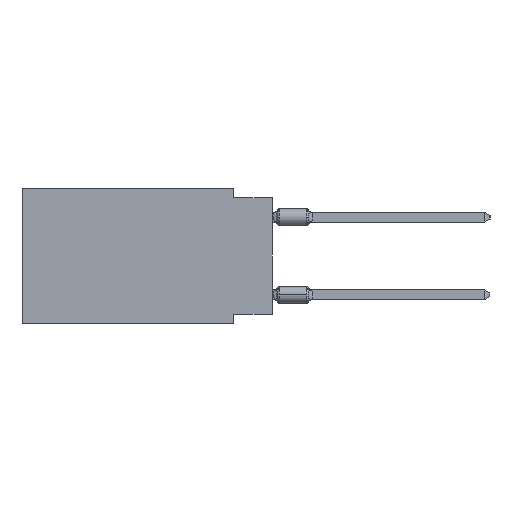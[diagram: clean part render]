
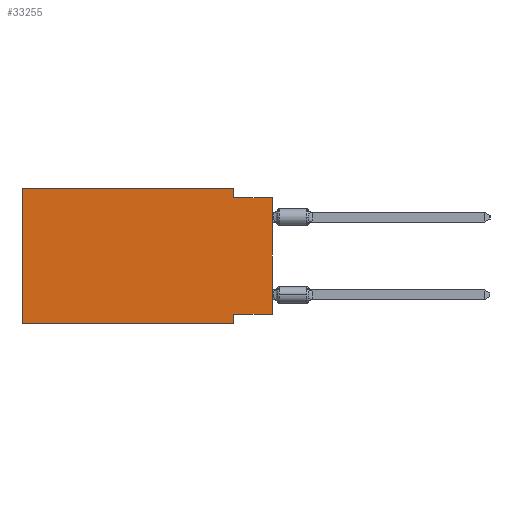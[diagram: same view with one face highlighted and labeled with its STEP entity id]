
A CAD part, left-side view. The second image highlights one B-rep face of the part: STEP entity #33255.
In plain terms, the highlighted planar face has unit normal (-1, 0, 0).
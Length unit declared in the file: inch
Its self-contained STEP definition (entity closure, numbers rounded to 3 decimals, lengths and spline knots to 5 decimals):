
#394 = CARTESIAN_POINT ( 'NONE',  ( 0., 0., -0.025 ) ) ;
#1127 = VERTEX_POINT ( 'NONE', #8704 ) ;
#1514 = EDGE_CURVE ( 'NONE', #1127, #52534, #60189, .T. ) ;
#3467 = VECTOR ( 'NONE', #20950, 39.37008 ) ;
#5479 = DIRECTION ( 'NONE',  ( 0., 0., -1. ) ) ;
#6096 = VECTOR ( 'NONE', #8203, 39.37008 ) ;
#6951 = EDGE_CURVE ( 'NONE', #21012, #21670, #28634, .T. ) ;
#8203 = DIRECTION ( 'NONE',  ( 0., 1., 0. ) ) ;
#8367 = CARTESIAN_POINT ( 'NONE',  ( 0., 0.1, -0.325 ) ) ;
#8704 = CARTESIAN_POINT ( 'NONE',  ( 0., 0.645, -0.35 ) ) ;
#10356 = VECTOR ( 'NONE', #22928, 39.37008 ) ;
#10448 = CARTESIAN_POINT ( 'NONE',  ( 0., 0.1, -0.35 ) ) ;
#11042 = DIRECTION ( 'NONE',  ( 0., 0., 1. ) ) ;
#12206 = AXIS2_PLACEMENT_3D ( 'NONE', #23310, #42154, #46177 ) ;
#14205 = CARTESIAN_POINT ( 'NONE',  ( 0., 0.645, 0. ) ) ;
#14236 = CARTESIAN_POINT ( 'NONE',  ( 0., 0.1, -0.025 ) ) ;
#14280 = LINE ( 'NONE', #47013, #35653 ) ;
#14366 = CARTESIAN_POINT ( 'NONE',  ( 0., 0., -0.325 ) ) ;
#16509 = VERTEX_POINT ( 'NONE', #33156 ) ;
#16996 = VECTOR ( 'NONE', #11042, 39.37008 ) ;
#17988 = LINE ( 'NONE', #18293, #10356 ) ;
#18278 = LINE ( 'NONE', #394, #33300 ) ;
#18293 = CARTESIAN_POINT ( 'NONE',  ( 0., 0.1, 0. ) ) ;
#18738 = ORIENTED_EDGE ( 'NONE', *, *, #6951, .F. ) ;
#20277 = CARTESIAN_POINT ( 'NONE',  ( 0., 0., 0. ) ) ;
#20950 = DIRECTION ( 'NONE',  ( 0., -1., 0. ) ) ;
#21012 = VERTEX_POINT ( 'NONE', #8367 ) ;
#21670 = VERTEX_POINT ( 'NONE', #10448 ) ;
#22928 = DIRECTION ( 'NONE',  ( 0., 0., -1. ) ) ;
#23310 = CARTESIAN_POINT ( 'NONE',  ( 0., 0.645, 0. ) ) ;
#24103 = ORIENTED_EDGE ( 'NONE', *, *, #29316, .F. ) ;
#27250 = DIRECTION ( 'NONE',  ( 0., -1., 0. ) ) ;
#28634 = LINE ( 'NONE', #37590, #31417 ) ;
#29156 = ORIENTED_EDGE ( 'NONE', *, *, #45169, .F. ) ;
#29316 = EDGE_CURVE ( 'NONE', #16509, #50217, #17988, .T. ) ;
#29779 = EDGE_CURVE ( 'NONE', #52534, #16509, #30245, .T. ) ;
#30245 = LINE ( 'NONE', #49066, #3467 ) ;
#31417 = VECTOR ( 'NONE', #5479, 39.37008 ) ;
#31975 = EDGE_CURVE ( 'NONE', #50217, #37402, #18278, .T. ) ;
#33089 = VERTEX_POINT ( 'NONE', #40033 ) ;
#33156 = CARTESIAN_POINT ( 'NONE',  ( 0., 0.1, 0. ) ) ;
#33255 = ADVANCED_FACE ( 'NONE', ( #46798 ), #50501, .F. ) ;
#33300 = VECTOR ( 'NONE', #46704, 39.37008 ) ;
#35653 = VECTOR ( 'NONE', #27250, 39.37008 ) ;
#37402 = VERTEX_POINT ( 'NONE', #55122 ) ;
#37590 = CARTESIAN_POINT ( 'NONE',  ( 0., 0.1, -0.35 ) ) ;
#37652 = VECTOR ( 'NONE', #37994, 39.37008 ) ;
#37994 = DIRECTION ( 'NONE',  ( 0., 0., 1. ) ) ;
#38781 = ORIENTED_EDGE ( 'NONE', *, *, #45988, .T. ) ;
#39331 = CARTESIAN_POINT ( 'NONE',  ( 0., 0.645, 0. ) ) ;
#40033 = CARTESIAN_POINT ( 'NONE',  ( 0., 0., -0.325 ) ) ;
#41865 = EDGE_LOOP ( 'NONE', ( #38781, #49825, #24103, #50135, #45831, #54717, #18738, #29156 ) ) ;
#42154 = DIRECTION ( 'NONE',  ( 1., 0., 0. ) ) ;
#43452 = EDGE_CURVE ( 'NONE', #1127, #21670, #14280, .T. ) ;
#45169 = EDGE_CURVE ( 'NONE', #33089, #21012, #56679, .T. ) ;
#45831 = ORIENTED_EDGE ( 'NONE', *, *, #1514, .F. ) ;
#45988 = EDGE_CURVE ( 'NONE', #33089, #37402, #53657, .T. ) ;
#46177 = DIRECTION ( 'NONE',  ( 0., 0., -1. ) ) ;
#46704 = DIRECTION ( 'NONE',  ( 0., -1., 0. ) ) ;
#46798 = FACE_OUTER_BOUND ( 'NONE', #41865, .T. ) ;
#47013 = CARTESIAN_POINT ( 'NONE',  ( 0., 0.645, -0.35 ) ) ;
#49066 = CARTESIAN_POINT ( 'NONE',  ( 0., 0.645, 0. ) ) ;
#49825 = ORIENTED_EDGE ( 'NONE', *, *, #31975, .F. ) ;
#50135 = ORIENTED_EDGE ( 'NONE', *, *, #29779, .F. ) ;
#50217 = VERTEX_POINT ( 'NONE', #14236 ) ;
#50501 = PLANE ( 'NONE',  #12206 ) ;
#52534 = VERTEX_POINT ( 'NONE', #39331 ) ;
#53657 = LINE ( 'NONE', #20277, #16996 ) ;
#54717 = ORIENTED_EDGE ( 'NONE', *, *, #43452, .T. ) ;
#55122 = CARTESIAN_POINT ( 'NONE',  ( 0., 0., -0.025 ) ) ;
#56679 = LINE ( 'NONE', #14366, #6096 ) ;
#60189 = LINE ( 'NONE', #14205, #37652 ) ;
